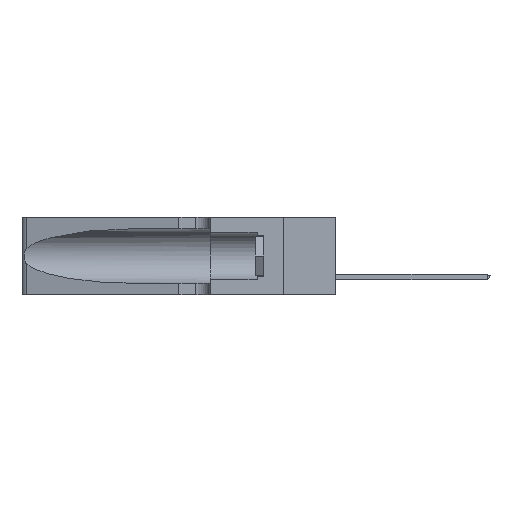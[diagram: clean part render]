
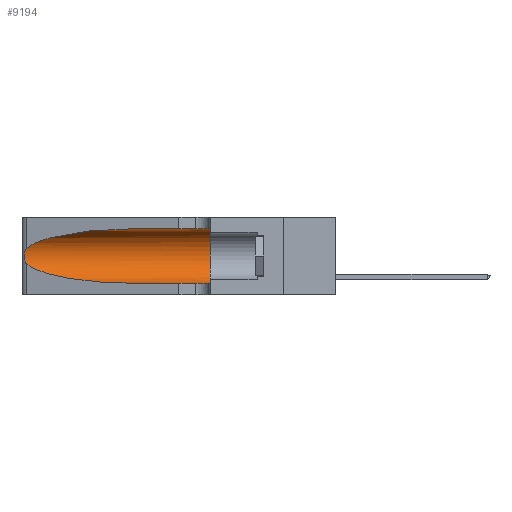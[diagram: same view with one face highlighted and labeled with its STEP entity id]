
A CAD part, left-side view. The second image highlights one B-rep face of the part: STEP entity #9194.
In plain terms, the highlighted cylindrical face has radius 3.308 mm (diameter 6.617 mm), a partial arc.
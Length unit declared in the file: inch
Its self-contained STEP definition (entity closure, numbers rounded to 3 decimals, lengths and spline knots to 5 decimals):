
#70 = CARTESIAN_POINT ( 'NONE',  ( 0.18966, 0.96281, 0.05475 ) ) ;
#596 = EDGE_CURVE ( 'NONE', #10308, #27576, #10013, .T. ) ;
#1025 = CARTESIAN_POINT ( 'NONE',  ( 0.1305, 0.72297, 0.31525 ) ) ;
#1826 = ORIENTED_EDGE ( 'NONE', *, *, #17861, .F. ) ;
#2188 = CIRCLE ( 'NONE', #31957, 0.13025 ) ;
#2914 = CARTESIAN_POINT ( 'NONE',  ( 0.2373, 1.15595, 0.08982 ) ) ;
#3701 = CARTESIAN_POINT ( 'NONE',  ( 0.25555, 1.22993, 0.14849 ) ) ;
#3813 = CARTESIAN_POINT ( 'NONE',  ( 0.26075, 1.23896, 0.178 ) ) ;
#3924 = CARTESIAN_POINT ( 'NONE',  ( 0.26018, 1.23835, 0.19895 ) ) ;
#3993 = ORIENTED_EDGE ( 'NONE', *, *, #596, .T. ) ;
#5587 = CARTESIAN_POINT ( 'NONE',  ( 0.1305, 0.35, 0.05475 ) ) ;
#5712 = DIRECTION ( 'NONE',  ( 0., -1., 0. ) ) ;
#5944 = DIRECTION ( 'NONE',  ( 0., 0., -1. ) ) ;
#6230 = CARTESIAN_POINT ( 'NONE',  ( 0.1305, 0.35, 0.185 ) ) ;
#6459 = CARTESIAN_POINT ( 'NONE',  ( 0.25639, 1.23184, 0.21858 ) ) ;
#7473 = ORIENTED_EDGE ( 'NONE', *, *, #9346, .F. ) ;
#7774 = CARTESIAN_POINT ( 'NONE',  ( 0.1305, 0.72297, 0.31525 ) ) ;
#7874 = VERTEX_POINT ( 'NONE', #25693 ) ;
#9020 = CARTESIAN_POINT ( 'NONE',  ( 0.25789, 1.23486, 0.15765 ) ) ;
#9194 = ADVANCED_FACE ( 'NONE', ( #14800 ), #12808, .F. ) ;
#9346 = EDGE_CURVE ( 'NONE', #11311, #7874, #12038, .T. ) ;
#9593 = EDGE_CURVE ( 'NONE', #30360, #10308, #15250, .T. ) ;
#9692 = DIRECTION ( 'NONE',  ( 0., -1., 0. ) ) ;
#10013 =( BOUNDED_CURVE ( )  B_SPLINE_CURVE ( 3, ( #15146, #2914, #70, #17612 ),
 .UNSPECIFIED., .F., .F. ) 
 B_SPLINE_CURVE_WITH_KNOTS ( ( 4, 4 ),
 ( 3.44316, 4.71239 ),
 .UNSPECIFIED. ) 
 CURVE ( )  GEOMETRIC_REPRESENTATION_ITEM ( )  RATIONAL_B_SPLINE_CURVE ( ( 1., 0.87, 0.87, 1. ) ) 
 REPRESENTATION_ITEM ( '' )  );
#10308 = VERTEX_POINT ( 'NONE', #31170 ) ;
#10411 = CARTESIAN_POINT ( 'NONE',  ( 0.18966, 0.96281, 0.31525 ) ) ;
#10770 = CARTESIAN_POINT ( 'NONE',  ( 0.1305, 1.61858, 0.05475 ) ) ;
#11311 = VERTEX_POINT ( 'NONE', #1025 ) ;
#12038 = LINE ( 'NONE', #22048, #17799 ) ;
#12170 = ORIENTED_EDGE ( 'NONE', *, *, #14551, .T. ) ;
#12808 = CYLINDRICAL_SURFACE ( 'NONE', #20293, 0.13025 ) ;
#14551 = EDGE_CURVE ( 'NONE', #11311, #30360, #31374, .T. ) ;
#14800 = FACE_OUTER_BOUND ( 'NONE', #25866, .T. ) ;
#15146 = CARTESIAN_POINT ( 'NONE',  ( 0.25487, 1.22718, 0.14631 ) ) ;
#15250 = B_SPLINE_CURVE_WITH_KNOTS ( 'NONE', 3,
 ( #18601, #31195, #6459, #21024, #23800, #3924, #28756, #3813, #16346, #16122, #9020, #28882, #3701, #21363 ),
 .UNSPECIFIED., .F., .F.,
 ( 4, 2, 2, 2, 2, 2, 4 ),
 ( 0., 0.00027, 0.00053, 0.00107, 0.0016, 0.00187, 0.00214 ),
 .UNSPECIFIED. ) ;
#16060 = CARTESIAN_POINT ( 'NONE',  ( 0.1305, 0.72297, 0.05475 ) ) ;
#16122 = CARTESIAN_POINT ( 'NONE',  ( 0.25856, 1.23593, 0.16098 ) ) ;
#16215 = DIRECTION ( 'NONE',  ( 0., 1., 0. ) ) ;
#16346 = CARTESIAN_POINT ( 'NONE',  ( 0.26017, 1.23833, 0.17102 ) ) ;
#17151 = ORIENTED_EDGE ( 'NONE', *, *, #17576, .T. ) ;
#17576 = EDGE_CURVE ( 'NONE', #27576, #20050, #30716, .T. ) ;
#17612 = CARTESIAN_POINT ( 'NONE',  ( 0.1305, 0.72297, 0.05475 ) ) ;
#17799 = VECTOR ( 'NONE', #9692, 39.37008 ) ;
#17861 = EDGE_CURVE ( 'NONE', #7874, #20050, #2188, .T. ) ;
#18601 = CARTESIAN_POINT ( 'NONE',  ( 0.25487, 1.22718, 0.22369 ) ) ;
#20050 = VERTEX_POINT ( 'NONE', #5587 ) ;
#20293 = AXIS2_PLACEMENT_3D ( 'NONE', #30918, #5712, #5944 ) ;
#21024 = CARTESIAN_POINT ( 'NONE',  ( 0.25787, 1.23484, 0.2124 ) ) ;
#21363 = CARTESIAN_POINT ( 'NONE',  ( 0.25487, 1.22718, 0.14631 ) ) ;
#22048 = CARTESIAN_POINT ( 'NONE',  ( 0.1305, 1.61858, 0.31525 ) ) ;
#23785 = DIRECTION ( 'NONE',  ( 0., 0., 1. ) ) ;
#23800 = CARTESIAN_POINT ( 'NONE',  ( 0.25854, 1.2359, 0.20912 ) ) ;
#24442 = VECTOR ( 'NONE', #25457, 39.37008 ) ;
#25457 = DIRECTION ( 'NONE',  ( 0., -1., 0. ) ) ;
#25693 = CARTESIAN_POINT ( 'NONE',  ( 0.1305, 0.35, 0.31525 ) ) ;
#25866 = EDGE_LOOP ( 'NONE', ( #12170, #29624, #3993, #17151, #1826, #7473 ) ) ;
#27576 = VERTEX_POINT ( 'NONE', #16060 ) ;
#27969 = CARTESIAN_POINT ( 'NONE',  ( 0.25487, 1.22718, 0.22369 ) ) ;
#28756 = CARTESIAN_POINT ( 'NONE',  ( 0.26075, 1.23896, 0.19203 ) ) ;
#28882 = CARTESIAN_POINT ( 'NONE',  ( 0.25639, 1.23186, 0.15144 ) ) ;
#29624 = ORIENTED_EDGE ( 'NONE', *, *, #9593, .T. ) ;
#30317 = CARTESIAN_POINT ( 'NONE',  ( 0.25487, 1.22718, 0.22369 ) ) ;
#30360 = VERTEX_POINT ( 'NONE', #30317 ) ;
#30631 = CARTESIAN_POINT ( 'NONE',  ( 0.2373, 1.15595, 0.28018 ) ) ;
#30716 = LINE ( 'NONE', #10770, #24442 ) ;
#30918 = CARTESIAN_POINT ( 'NONE',  ( 0.1305, 1.61858, 0.185 ) ) ;
#31170 = CARTESIAN_POINT ( 'NONE',  ( 0.25487, 1.22718, 0.14631 ) ) ;
#31195 = CARTESIAN_POINT ( 'NONE',  ( 0.25555, 1.22994, 0.2215 ) ) ;
#31374 =( BOUNDED_CURVE ( )  B_SPLINE_CURVE ( 3, ( #7774, #10411, #30631, #27969 ),
 .UNSPECIFIED., .F., .T. ) 
 B_SPLINE_CURVE_WITH_KNOTS ( ( 4, 4 ),
 ( 1.5708, 2.84003 ),
 .UNSPECIFIED. ) 
 CURVE ( )  GEOMETRIC_REPRESENTATION_ITEM ( )  RATIONAL_B_SPLINE_CURVE ( ( 1., 0.87, 0.87, 1. ) ) 
 REPRESENTATION_ITEM ( '' )  );
#31957 = AXIS2_PLACEMENT_3D ( 'NONE', #6230, #16215, #23785 ) ;
